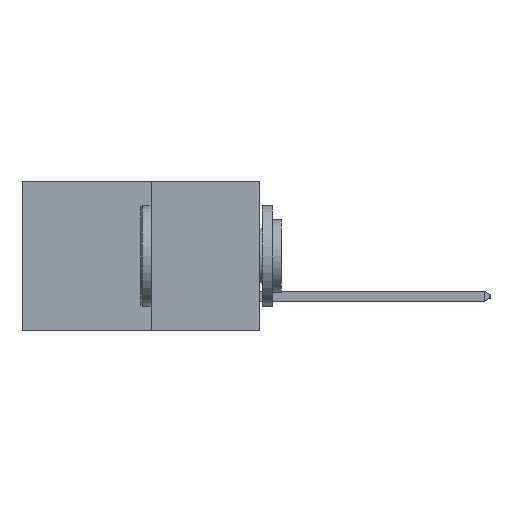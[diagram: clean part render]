
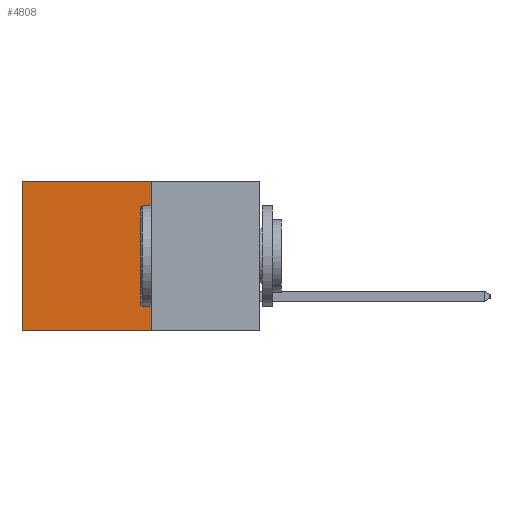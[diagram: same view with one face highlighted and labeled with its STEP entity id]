
A CAD part, left-side view. The second image highlights one B-rep face of the part: STEP entity #4808.
In plain terms, the highlighted planar face has unit normal (-1, 0, 0).
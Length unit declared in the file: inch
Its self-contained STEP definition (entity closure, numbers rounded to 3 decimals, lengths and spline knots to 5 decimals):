
#60 = VERTEX_POINT ( 'NONE', #1313 ) ;
#726 = DIRECTION ( 'NONE',  ( 0., 0., -1. ) ) ;
#804 = DIRECTION ( 'NONE',  ( 1., 0., 0. ) ) ;
#874 = PLANE ( 'NONE',  #2889 ) ;
#1057 = CARTESIAN_POINT ( 'NONE',  ( 0.277, 0.27, -0.37 ) ) ;
#1066 = VERTEX_POINT ( 'NONE', #7447 ) ;
#1313 = CARTESIAN_POINT ( 'NONE',  ( 0.277, 0.27, 0. ) ) ;
#1531 = EDGE_CURVE ( 'NONE', #1066, #15389, #3098, .T. ) ;
#2158 = ORIENTED_EDGE ( 'NONE', *, *, #13087, .F. ) ;
#2703 = CARTESIAN_POINT ( 'NONE',  ( 0.277, 0.27, -0.37 ) ) ;
#2889 = AXIS2_PLACEMENT_3D ( 'NONE', #1057, #804, #726 ) ;
#3098 = LINE ( 'NONE', #12691, #16247 ) ;
#4635 = CARTESIAN_POINT ( 'NONE',  ( 0.277, 0.59, -0.37 ) ) ;
#4712 = VECTOR ( 'NONE', #13403, 39.37008 ) ;
#4808 = ADVANCED_FACE ( 'NONE', ( #16046 ), #874, .F. ) ;
#5226 = LINE ( 'NONE', #4635, #17772 ) ;
#5540 = CARTESIAN_POINT ( 'NONE',  ( 0.277, 0.59, -0.37 ) ) ;
#7447 = CARTESIAN_POINT ( 'NONE',  ( 0.277, 0.27, -0.37 ) ) ;
#7865 = VERTEX_POINT ( 'NONE', #8287 ) ;
#7928 = ORIENTED_EDGE ( 'NONE', *, *, #1531, .F. ) ;
#8287 = CARTESIAN_POINT ( 'NONE',  ( 0.277, 0.59, 0. ) ) ;
#10116 = CARTESIAN_POINT ( 'NONE',  ( 0.277, 0.27, 0. ) ) ;
#11267 = EDGE_CURVE ( 'NONE', #60, #7865, #17783, .T. ) ;
#12144 = DIRECTION ( 'NONE',  ( 0., 1., 0. ) ) ;
#12691 = CARTESIAN_POINT ( 'NONE',  ( 0.277, 0.27, -0.37 ) ) ;
#13087 = EDGE_CURVE ( 'NONE', #60, #1066, #19768, .T. ) ;
#13403 = DIRECTION ( 'NONE',  ( 0., 1., 0. ) ) ;
#14244 = DIRECTION ( 'NONE',  ( 0., 0., -1. ) ) ;
#14435 = EDGE_CURVE ( 'NONE', #7865, #15389, #5226, .T. ) ;
#15389 = VERTEX_POINT ( 'NONE', #5540 ) ;
#16046 = FACE_OUTER_BOUND ( 'NONE', #19526, .T. ) ;
#16072 = DIRECTION ( 'NONE',  ( 0., 0., -1. ) ) ;
#16247 = VECTOR ( 'NONE', #12144, 39.37008 ) ;
#17772 = VECTOR ( 'NONE', #16072, 39.37008 ) ;
#17783 = LINE ( 'NONE', #10116, #4712 ) ;
#17896 = ORIENTED_EDGE ( 'NONE', *, *, #14435, .T. ) ;
#19526 = EDGE_LOOP ( 'NONE', ( #17896, #7928, #2158, #19987 ) ) ;
#19768 = LINE ( 'NONE', #2703, #20275 ) ;
#19987 = ORIENTED_EDGE ( 'NONE', *, *, #11267, .T. ) ;
#20275 = VECTOR ( 'NONE', #14244, 39.37008 ) ;
